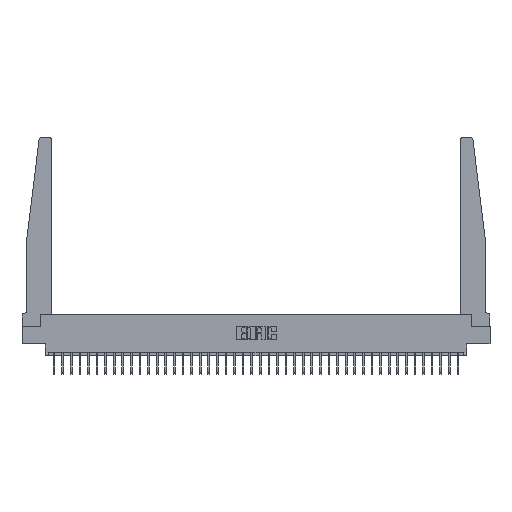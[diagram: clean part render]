
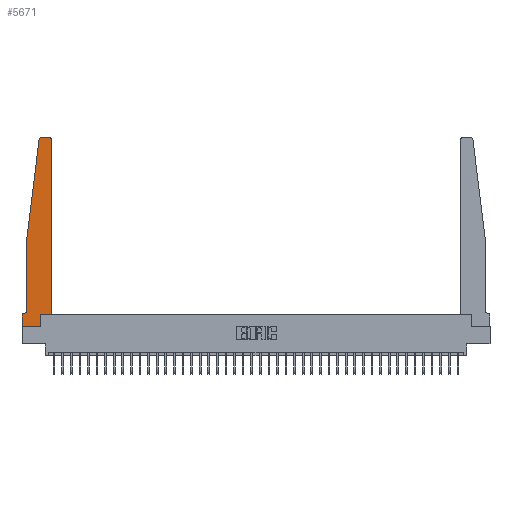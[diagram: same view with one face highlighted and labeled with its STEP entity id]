
A CAD part, top view. The second image highlights one B-rep face of the part: STEP entity #5671.
In plain terms, the highlighted planar face has unit normal (0, 0, 1).
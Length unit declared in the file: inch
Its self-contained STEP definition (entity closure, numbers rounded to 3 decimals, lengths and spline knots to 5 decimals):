
#53 = CARTESIAN_POINT ( 'NONE',  ( 0., 0.1875, 0.37 ) ) ;
#576 = DIRECTION ( 'NONE',  ( 0., 0., 1. ) ) ;
#805 = VERTEX_POINT ( 'NONE', #14520 ) ;
#918 = EDGE_CURVE ( 'NONE', #7422, #805, #13316, .T. ) ;
#1017 = CARTESIAN_POINT ( 'NONE',  ( 0.425, 2.72, 0.37 ) ) ;
#1176 = CARTESIAN_POINT ( 'NONE',  ( 0.395, 2.75, 0.37 ) ) ;
#2097 = EDGE_CURVE ( 'NONE', #6765, #22948, #19064, .T. ) ;
#2431 = VECTOR ( 'NONE', #2739, 39.37008 ) ;
#2529 = CARTESIAN_POINT ( 'NONE',  ( 0.065, 1.25, 0.37 ) ) ;
#2739 = DIRECTION ( 'NONE',  ( -0.122, -0.992, 0. ) ) ;
#3020 = CARTESIAN_POINT ( 'NONE',  ( 0.25, 2.75, 0.37 ) ) ;
#3123 = VERTEX_POINT ( 'NONE', #2529 ) ;
#3249 = CARTESIAN_POINT ( 'NONE',  ( 0.015, 0.1875, 0.37 ) ) ;
#4316 = DIRECTION ( 'NONE',  ( 0., 0., -1. ) ) ;
#4340 = CARTESIAN_POINT ( 'NONE',  ( 0., 0.1875, 0.37 ) ) ;
#4712 = PLANE ( 'NONE',  #32297 ) ;
#5054 = VERTEX_POINT ( 'NONE', #18331 ) ;
#5343 = EDGE_CURVE ( 'NONE', #13531, #25492, #29256, .T. ) ;
#5671 = ADVANCED_FACE ( 'NONE', ( #30270 ), #4712, .T. ) ;
#6306 = CARTESIAN_POINT ( 'NONE',  ( 0.27653, 2.72, 0.37 ) ) ;
#6671 = VECTOR ( 'NONE', #21246, 39.37008 ) ;
#6761 = LINE ( 'NONE', #18600, #21777 ) ;
#6765 = VERTEX_POINT ( 'NONE', #27950 ) ;
#6986 = VECTOR ( 'NONE', #26299, 39.37008 ) ;
#7422 = VERTEX_POINT ( 'NONE', #17995 ) ;
#7500 = VERTEX_POINT ( 'NONE', #35501 ) ;
#8846 = VECTOR ( 'NONE', #22674, 39.37008 ) ;
#9173 = AXIS2_PLACEMENT_3D ( 'NONE', #26099, #22874, #37147 ) ;
#9754 = DIRECTION ( 'NONE',  ( 0., -1., 0. ) ) ;
#10668 = ORIENTED_EDGE ( 'NONE', *, *, #34134, .T. ) ;
#10840 = CARTESIAN_POINT ( 'NONE',  ( 0.425, 0.18, 0.37 ) ) ;
#11580 = ORIENTED_EDGE ( 'NONE', *, *, #17151, .T. ) ;
#11624 = CARTESIAN_POINT ( 'NONE',  ( 0.2605, 0., 0.37 ) ) ;
#11686 = DIRECTION ( 'NONE',  ( -1., 0., 0. ) ) ;
#12218 = DIRECTION ( 'NONE',  ( 1., 0., 0. ) ) ;
#12224 = EDGE_LOOP ( 'NONE', ( #20542, #25275, #18091, #33947, #11580, #35823, #36198, #10668, #15968, #13388, #30780, #31126 ) ) ;
#12813 = LINE ( 'NONE', #24423, #34672 ) ;
#12857 = CARTESIAN_POINT ( 'NONE',  ( 0., 0., 0.37 ) ) ;
#13316 = CIRCLE ( 'NONE', #34576, 0.03 ) ;
#13388 = ORIENTED_EDGE ( 'NONE', *, *, #2097, .T. ) ;
#13531 = VERTEX_POINT ( 'NONE', #1017 ) ;
#13535 = VECTOR ( 'NONE', #14545, 39.37008 ) ;
#13587 = EDGE_CURVE ( 'NONE', #20767, #7500, #20871, .T. ) ;
#14173 = LINE ( 'NONE', #20265, #13535 ) ;
#14520 = CARTESIAN_POINT ( 'NONE',  ( 0.24675, 2.72367, 0.37 ) ) ;
#14545 = DIRECTION ( 'NONE',  ( 0., 1., 0. ) ) ;
#14821 = EDGE_CURVE ( 'NONE', #805, #3123, #34956, .T. ) ;
#15968 = ORIENTED_EDGE ( 'NONE', *, *, #25096, .T. ) ;
#16677 = EDGE_CURVE ( 'NONE', #22948, #13531, #14173, .T. ) ;
#17151 = EDGE_CURVE ( 'NONE', #5054, #37300, #24524, .T. ) ;
#17995 = CARTESIAN_POINT ( 'NONE',  ( 0.27653, 2.75, 0.37 ) ) ;
#18036 = DIRECTION ( 'NONE',  ( 0., 1., 0. ) ) ;
#18091 = ORIENTED_EDGE ( 'NONE', *, *, #14821, .T. ) ;
#18108 = EDGE_CURVE ( 'NONE', #3123, #5054, #35682, .T. ) ;
#18331 = CARTESIAN_POINT ( 'NONE',  ( 0.065, 0.2375, 0.37 ) ) ;
#18600 = CARTESIAN_POINT ( 'NONE',  ( 0.2605, 0.18, 0.37 ) ) ;
#19064 = LINE ( 'NONE', #10840, #8846 ) ;
#20265 = CARTESIAN_POINT ( 'NONE',  ( 0.425, 0.18, 0.37 ) ) ;
#20542 = ORIENTED_EDGE ( 'NONE', *, *, #26949, .T. ) ;
#20767 = VERTEX_POINT ( 'NONE', #53 ) ;
#20871 = LINE ( 'NONE', #12857, #6671 ) ;
#21246 = DIRECTION ( 'NONE',  ( 0., -1., 0. ) ) ;
#21484 = AXIS2_PLACEMENT_3D ( 'NONE', #21864, #4316, #24715 ) ;
#21777 = VECTOR ( 'NONE', #18036, 39.37008 ) ;
#21864 = CARTESIAN_POINT ( 'NONE',  ( 0.015, 0.2375, 0.37 ) ) ;
#22674 = DIRECTION ( 'NONE',  ( 1., 0., 0. ) ) ;
#22874 = DIRECTION ( 'NONE',  ( 0., 0., 1. ) ) ;
#22948 = VERTEX_POINT ( 'NONE', #33139 ) ;
#24423 = CARTESIAN_POINT ( 'NONE',  ( 0., 0., 0.37 ) ) ;
#24524 = CIRCLE ( 'NONE', #21484, 0.05 ) ;
#24549 = VECTOR ( 'NONE', #9754, 39.37008 ) ;
#24715 = DIRECTION ( 'NONE',  ( -1., 0., 0. ) ) ;
#25096 = EDGE_CURVE ( 'NONE', #26846, #6765, #6761, .T. ) ;
#25275 = ORIENTED_EDGE ( 'NONE', *, *, #918, .T. ) ;
#25315 = EDGE_CURVE ( 'NONE', #37300, #20767, #33986, .T. ) ;
#25492 = VERTEX_POINT ( 'NONE', #1176 ) ;
#26099 = CARTESIAN_POINT ( 'NONE',  ( 0.395, 2.72, 0.37 ) ) ;
#26111 = LINE ( 'NONE', #3020, #6986 ) ;
#26299 = DIRECTION ( 'NONE',  ( -1., 0., 0. ) ) ;
#26846 = VERTEX_POINT ( 'NONE', #11624 ) ;
#26949 = EDGE_CURVE ( 'NONE', #25492, #7422, #26111, .T. ) ;
#27404 = DIRECTION ( 'NONE',  ( 0., 0., 1. ) ) ;
#27950 = CARTESIAN_POINT ( 'NONE',  ( 0.2605, 0.18, 0.37 ) ) ;
#28375 = VECTOR ( 'NONE', #11686, 39.37008 ) ;
#29256 = CIRCLE ( 'NONE', #9173, 0.03 ) ;
#30148 = CARTESIAN_POINT ( 'NONE',  ( 0.065, 1.25, 0.37 ) ) ;
#30270 = FACE_OUTER_BOUND ( 'NONE', #12224, .T. ) ;
#30780 = ORIENTED_EDGE ( 'NONE', *, *, #16677, .T. ) ;
#31126 = ORIENTED_EDGE ( 'NONE', *, *, #5343, .T. ) ;
#32063 = CARTESIAN_POINT ( 'NONE',  ( 0.065, 0.1875, 0.37 ) ) ;
#32297 = AXIS2_PLACEMENT_3D ( 'NONE', #4340, #27404, #33492 ) ;
#33139 = CARTESIAN_POINT ( 'NONE',  ( 0.425, 0.18, 0.37 ) ) ;
#33492 = DIRECTION ( 'NONE',  ( 1., 0., 0. ) ) ;
#33947 = ORIENTED_EDGE ( 'NONE', *, *, #18108, .T. ) ;
#33986 = LINE ( 'NONE', #32063, #28375 ) ;
#34134 = EDGE_CURVE ( 'NONE', #7500, #26846, #12813, .T. ) ;
#34576 = AXIS2_PLACEMENT_3D ( 'NONE', #6306, #576, #12218 ) ;
#34672 = VECTOR ( 'NONE', #36046, 39.37008 ) ;
#34956 = LINE ( 'NONE', #37626, #2431 ) ;
#35501 = CARTESIAN_POINT ( 'NONE',  ( 0., 0., 0.37 ) ) ;
#35682 = LINE ( 'NONE', #30148, #24549 ) ;
#35823 = ORIENTED_EDGE ( 'NONE', *, *, #25315, .T. ) ;
#36046 = DIRECTION ( 'NONE',  ( 1., 0., 0. ) ) ;
#36198 = ORIENTED_EDGE ( 'NONE', *, *, #13587, .T. ) ;
#37147 = DIRECTION ( 'NONE',  ( 1., 0., 0. ) ) ;
#37300 = VERTEX_POINT ( 'NONE', #3249 ) ;
#37626 = CARTESIAN_POINT ( 'NONE',  ( 0.065, 1.25, 0.37 ) ) ;
